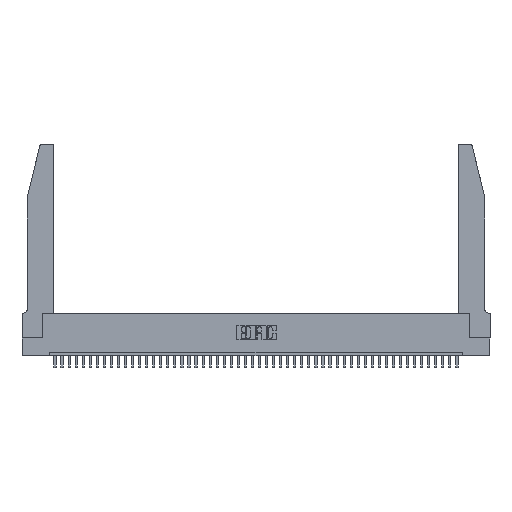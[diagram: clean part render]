
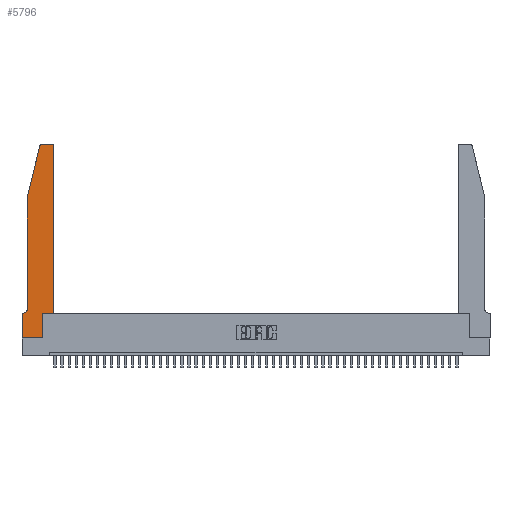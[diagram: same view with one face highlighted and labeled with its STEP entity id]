
A CAD part, top view. The second image highlights one B-rep face of the part: STEP entity #5796.
In plain terms, the highlighted planar face has unit normal (0, 0, 1).
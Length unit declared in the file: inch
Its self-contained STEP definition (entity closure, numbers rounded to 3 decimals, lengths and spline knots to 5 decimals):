
#103 = EDGE_CURVE ( 'NONE', #32844, #36914, #45323, .T. ) ;
#1328 = ORIENTED_EDGE ( 'NONE', *, *, #23770, .T. ) ;
#1408 = VERTEX_POINT ( 'NONE', #29843 ) ;
#2426 = CARTESIAN_POINT ( 'NONE',  ( 0.284, 2.75, 0.37 ) ) ;
#2443 = VECTOR ( 'NONE', #16501, 39.37008 ) ;
#3424 = AXIS2_PLACEMENT_3D ( 'NONE', #21658, #43399, #39480 ) ;
#3528 = ORIENTED_EDGE ( 'NONE', *, *, #25525, .T. ) ;
#3882 = CARTESIAN_POINT ( 'NONE',  ( 0.2865, 0.35, 0.37 ) ) ;
#5283 = DIRECTION ( 'NONE',  ( 1., 0., 0. ) ) ;
#5796 = ADVANCED_FACE ( 'NONE', ( #40842 ), #11140, .T. ) ;
#6020 = CARTESIAN_POINT ( 'NONE',  ( 0.4205, 2.72, 0.37 ) ) ;
#6880 = VECTOR ( 'NONE', #34306, 39.37008 ) ;
#7252 = VERTEX_POINT ( 'NONE', #13914 ) ;
#7540 = ORIENTED_EDGE ( 'NONE', *, *, #35359, .T. ) ;
#7637 = ORIENTED_EDGE ( 'NONE', *, *, #27395, .T. ) ;
#8066 = EDGE_LOOP ( 'NONE', ( #16543, #14106, #3528, #8434, #1328, #15407, #7637, #27580, #21965, #27460, #7540, #38684 ) ) ;
#8434 = ORIENTED_EDGE ( 'NONE', *, *, #22073, .T. ) ;
#8451 = AXIS2_PLACEMENT_3D ( 'NONE', #9981, #16750, #23591 ) ;
#8550 = DIRECTION ( 'NONE',  ( 0., -1., 0. ) ) ;
#9132 = DIRECTION ( 'NONE',  ( 0., 0., 1. ) ) ;
#9379 = EDGE_CURVE ( 'NONE', #15562, #15551, #44545, .T. ) ;
#9972 = DIRECTION ( 'NONE',  ( -0.239, -0.971, 0. ) ) ;
#9981 = CARTESIAN_POINT ( 'NONE',  ( 0.0055, 0.42, 0.37 ) ) ;
#10137 = CARTESIAN_POINT ( 'NONE',  ( 0.0755, 2., 0.37 ) ) ;
#10237 = CIRCLE ( 'NONE', #20090, 0.03 ) ;
#10617 = VECTOR ( 'NONE', #29436, 39.37008 ) ;
#11140 = PLANE ( 'NONE',  #3424 ) ;
#13205 = VECTOR ( 'NONE', #30410, 39.37008 ) ;
#13332 = VECTOR ( 'NONE', #8550, 39.37008 ) ;
#13345 = CIRCLE ( 'NONE', #8451, 0.07 ) ;
#13914 = CARTESIAN_POINT ( 'NONE',  ( 0.2865, 0., 0.37 ) ) ;
#14106 = ORIENTED_EDGE ( 'NONE', *, *, #21934, .T. ) ;
#15407 = ORIENTED_EDGE ( 'NONE', *, *, #103, .T. ) ;
#15551 = VERTEX_POINT ( 'NONE', #2426 ) ;
#15562 = VERTEX_POINT ( 'NONE', #38456 ) ;
#15601 = CARTESIAN_POINT ( 'NONE',  ( 0.0755, 2., 0.37 ) ) ;
#16152 = CARTESIAN_POINT ( 'NONE',  ( 0.4505, 0.35, 0.37 ) ) ;
#16360 = EDGE_CURVE ( 'NONE', #42616, #29823, #24247, .T. ) ;
#16501 = DIRECTION ( 'NONE',  ( 0., 1., 0. ) ) ;
#16543 = ORIENTED_EDGE ( 'NONE', *, *, #9379, .T. ) ;
#16568 = CARTESIAN_POINT ( 'NONE',  ( 0.0755, 0.35, 0.37 ) ) ;
#16750 = DIRECTION ( 'NONE',  ( 0., 0., -1. ) ) ;
#16969 = VECTOR ( 'NONE', #28287, 39.37008 ) ;
#17146 = LINE ( 'NONE', #10137, #42327 ) ;
#17971 = VECTOR ( 'NONE', #22328, 39.37008 ) ;
#18591 = CARTESIAN_POINT ( 'NONE',  ( 0., 0., 0.37 ) ) ;
#18915 = CARTESIAN_POINT ( 'NONE',  ( 0.2605, 2.75, 0.37 ) ) ;
#20090 = AXIS2_PLACEMENT_3D ( 'NONE', #6020, #9132, #37456 ) ;
#20295 = EDGE_CURVE ( 'NONE', #1408, #7252, #21354, .T. ) ;
#21354 = LINE ( 'NONE', #18591, #17971 ) ;
#21658 = CARTESIAN_POINT ( 'NONE',  ( 0., 0.35, 0.37 ) ) ;
#21934 = EDGE_CURVE ( 'NONE', #15551, #38356, #45289, .T. ) ;
#21965 = ORIENTED_EDGE ( 'NONE', *, *, #38978, .T. ) ;
#22073 = EDGE_CURVE ( 'NONE', #40615, #39018, #32349, .T. ) ;
#22328 = DIRECTION ( 'NONE',  ( 1., 0., 0. ) ) ;
#23279 = DIRECTION ( 'NONE',  ( 0., 0., 1. ) ) ;
#23591 = DIRECTION ( 'NONE',  ( -1., 0., 0. ) ) ;
#23676 = LINE ( 'NONE', #30470, #16969 ) ;
#23770 = EDGE_CURVE ( 'NONE', #39018, #32844, #13345, .T. ) ;
#24247 = LINE ( 'NONE', #16152, #6880 ) ;
#25525 = EDGE_CURVE ( 'NONE', #38356, #40615, #17146, .T. ) ;
#25695 = LINE ( 'NONE', #25806, #10617 ) ;
#25806 = CARTESIAN_POINT ( 'NONE',  ( 0.2865, 0.35, 0.37 ) ) ;
#27395 = EDGE_CURVE ( 'NONE', #36914, #1408, #23676, .T. ) ;
#27460 = ORIENTED_EDGE ( 'NONE', *, *, #16360, .T. ) ;
#27580 = ORIENTED_EDGE ( 'NONE', *, *, #20295, .T. ) ;
#28280 = AXIS2_PLACEMENT_3D ( 'NONE', #37190, #23279, #5283 ) ;
#28287 = DIRECTION ( 'NONE',  ( 0., -1., 0. ) ) ;
#29436 = DIRECTION ( 'NONE',  ( 0., 1., 0. ) ) ;
#29823 = VERTEX_POINT ( 'NONE', #43097 ) ;
#29843 = CARTESIAN_POINT ( 'NONE',  ( 0., 0., 0.37 ) ) ;
#30012 = VERTEX_POINT ( 'NONE', #45163 ) ;
#30410 = DIRECTION ( 'NONE',  ( -1., 0., 0. ) ) ;
#30470 = CARTESIAN_POINT ( 'NONE',  ( 0., 0., 0.37 ) ) ;
#30566 = CARTESIAN_POINT ( 'NONE',  ( 0.4505, 0.35, 0.37 ) ) ;
#32349 = LINE ( 'NONE', #34239, #13332 ) ;
#32380 = VECTOR ( 'NONE', #41430, 39.37008 ) ;
#32844 = VERTEX_POINT ( 'NONE', #40748 ) ;
#34239 = CARTESIAN_POINT ( 'NONE',  ( 0.0755, 2., 0.37 ) ) ;
#34306 = DIRECTION ( 'NONE',  ( 1., 0., 0. ) ) ;
#35359 = EDGE_CURVE ( 'NONE', #29823, #30012, #41556, .T. ) ;
#36914 = VERTEX_POINT ( 'NONE', #38533 ) ;
#37068 = CARTESIAN_POINT ( 'NONE',  ( 0.0755, 0.42, 0.37 ) ) ;
#37190 = CARTESIAN_POINT ( 'NONE',  ( 0.284, 2.72, 0.37 ) ) ;
#37456 = DIRECTION ( 'NONE',  ( 1., 0., 0. ) ) ;
#38356 = VERTEX_POINT ( 'NONE', #39765 ) ;
#38456 = CARTESIAN_POINT ( 'NONE',  ( 0.4205, 2.75, 0.37 ) ) ;
#38533 = CARTESIAN_POINT ( 'NONE',  ( 0., 0.35, 0.37 ) ) ;
#38684 = ORIENTED_EDGE ( 'NONE', *, *, #45633, .T. ) ;
#38978 = EDGE_CURVE ( 'NONE', #7252, #42616, #25695, .T. ) ;
#39018 = VERTEX_POINT ( 'NONE', #37068 ) ;
#39480 = DIRECTION ( 'NONE',  ( 1., 0., 0. ) ) ;
#39765 = CARTESIAN_POINT ( 'NONE',  ( 0.25487, 2.72718, 0.37 ) ) ;
#40615 = VERTEX_POINT ( 'NONE', #15601 ) ;
#40748 = CARTESIAN_POINT ( 'NONE',  ( 0.0055, 0.35, 0.37 ) ) ;
#40842 = FACE_OUTER_BOUND ( 'NONE', #8066, .T. ) ;
#41430 = DIRECTION ( 'NONE',  ( -1., 0., 0. ) ) ;
#41556 = LINE ( 'NONE', #30566, #2443 ) ;
#42327 = VECTOR ( 'NONE', #9972, 39.37008 ) ;
#42616 = VERTEX_POINT ( 'NONE', #3882 ) ;
#43097 = CARTESIAN_POINT ( 'NONE',  ( 0.4505, 0.35, 0.37 ) ) ;
#43399 = DIRECTION ( 'NONE',  ( 0., 0., 1. ) ) ;
#44545 = LINE ( 'NONE', #18915, #13205 ) ;
#45163 = CARTESIAN_POINT ( 'NONE',  ( 0.4505, 2.72, 0.37 ) ) ;
#45289 = CIRCLE ( 'NONE', #28280, 0.03 ) ;
#45323 = LINE ( 'NONE', #16568, #32380 ) ;
#45633 = EDGE_CURVE ( 'NONE', #30012, #15562, #10237, .T. ) ;
